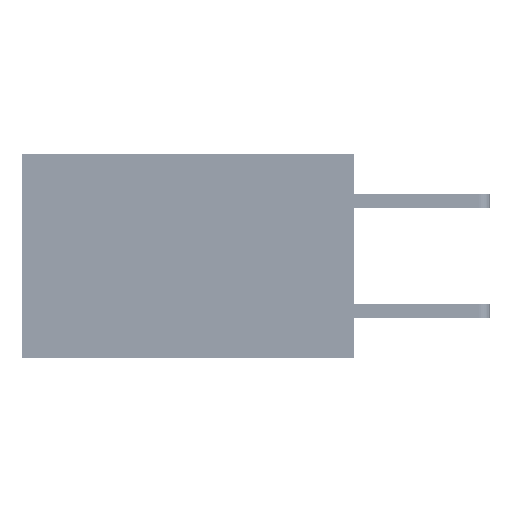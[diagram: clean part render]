
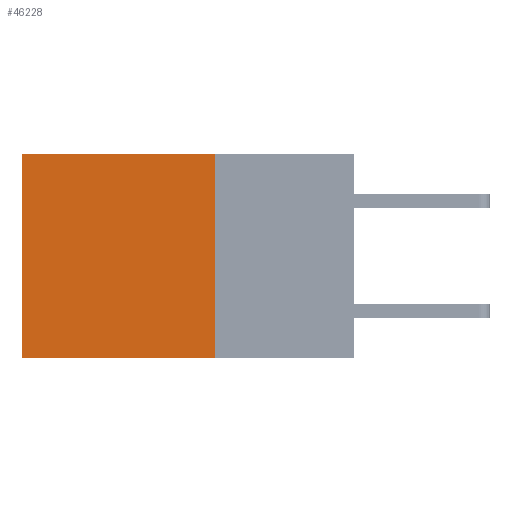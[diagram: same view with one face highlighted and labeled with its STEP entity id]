
A CAD part, left-side view. The second image highlights one B-rep face of the part: STEP entity #46228.
In plain terms, the highlighted planar face has unit normal (-1, 0, 0).
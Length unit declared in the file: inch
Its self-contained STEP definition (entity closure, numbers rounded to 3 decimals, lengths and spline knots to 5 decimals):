
#724 = VERTEX_POINT ( 'NONE', #33933 ) ;
#1242 = ORIENTED_EDGE ( 'NONE', *, *, #21212, .F. ) ;
#3457 = VECTOR ( 'NONE', #16621, 39.37008 ) ;
#4032 = ORIENTED_EDGE ( 'NONE', *, *, #49693, .T. ) ;
#5443 = DIRECTION ( 'NONE',  ( 0., 0., -1. ) ) ;
#6156 = LINE ( 'NONE', #9357, #24434 ) ;
#6393 = AXIS2_PLACEMENT_3D ( 'NONE', #27712, #16008, #27554 ) ;
#9357 = CARTESIAN_POINT ( 'NONE',  ( 0.2875, 0.6, 0. ) ) ;
#11563 = CARTESIAN_POINT ( 'NONE',  ( 0.2875, 0.25, -0.37 ) ) ;
#13174 = CARTESIAN_POINT ( 'NONE',  ( 0.2875, 0.25, -0.37 ) ) ;
#14096 = PLANE ( 'NONE',  #6393 ) ;
#16008 = DIRECTION ( 'NONE',  ( 1., 0., 0. ) ) ;
#16021 = CARTESIAN_POINT ( 'NONE',  ( 0.2875, 0.6, -0.37 ) ) ;
#16621 = DIRECTION ( 'NONE',  ( 0., 1., 0. ) ) ;
#16682 = EDGE_CURVE ( 'NONE', #724, #48332, #6156, .T. ) ;
#18021 = EDGE_CURVE ( 'NONE', #29349, #48332, #34506, .T. ) ;
#21212 = EDGE_CURVE ( 'NONE', #49900, #29349, #35489, .T. ) ;
#22947 = ORIENTED_EDGE ( 'NONE', *, *, #16682, .T. ) ;
#24434 = VECTOR ( 'NONE', #5443, 39.37008 ) ;
#27394 = CARTESIAN_POINT ( 'NONE',  ( 0.2875, 0.25, 0. ) ) ;
#27554 = DIRECTION ( 'NONE',  ( 0., 0., -1. ) ) ;
#27712 = CARTESIAN_POINT ( 'NONE',  ( 0.2875, 0.25, 0. ) ) ;
#29349 = VERTEX_POINT ( 'NONE', #11563 ) ;
#30906 = VECTOR ( 'NONE', #50389, 39.37008 ) ;
#33933 = CARTESIAN_POINT ( 'NONE',  ( 0.2875, 0.6, 0. ) ) ;
#34253 = VECTOR ( 'NONE', #37646, 39.37008 ) ;
#34506 = LINE ( 'NONE', #13174, #3457 ) ;
#35489 = LINE ( 'NONE', #45337, #34253 ) ;
#37646 = DIRECTION ( 'NONE',  ( 0., 0., -1. ) ) ;
#43722 = LINE ( 'NONE', #27394, #30906 ) ;
#44963 = CARTESIAN_POINT ( 'NONE',  ( 0.2875, 0.25, 0. ) ) ;
#45337 = CARTESIAN_POINT ( 'NONE',  ( 0.2875, 0.25, 0. ) ) ;
#45538 = FACE_OUTER_BOUND ( 'NONE', #50025, .T. ) ;
#46228 = ADVANCED_FACE ( 'NONE', ( #45538 ), #14096, .F. ) ;
#47802 = ORIENTED_EDGE ( 'NONE', *, *, #18021, .F. ) ;
#48332 = VERTEX_POINT ( 'NONE', #16021 ) ;
#49693 = EDGE_CURVE ( 'NONE', #49900, #724, #43722, .T. ) ;
#49900 = VERTEX_POINT ( 'NONE', #44963 ) ;
#50025 = EDGE_LOOP ( 'NONE', ( #22947, #47802, #1242, #4032 ) ) ;
#50389 = DIRECTION ( 'NONE',  ( 0., 1., 0. ) ) ;
